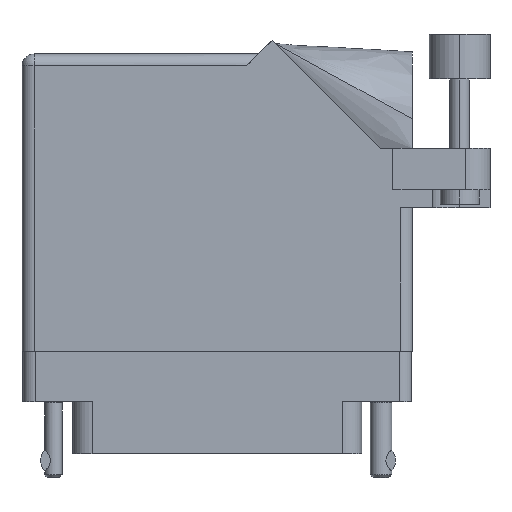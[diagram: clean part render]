
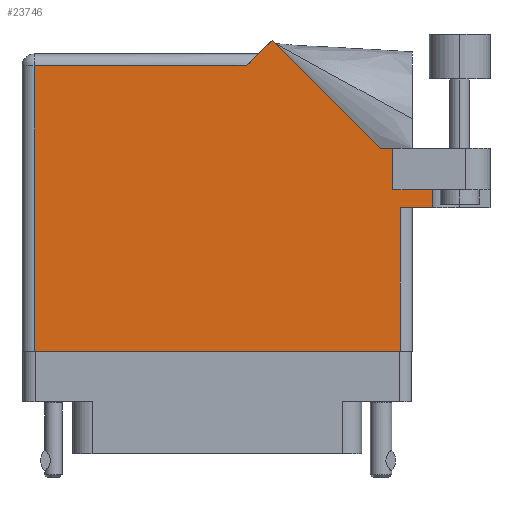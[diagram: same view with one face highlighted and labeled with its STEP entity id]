
A CAD part, front view. The second image highlights one B-rep face of the part: STEP entity #23746.
In plain terms, the highlighted face is planar.
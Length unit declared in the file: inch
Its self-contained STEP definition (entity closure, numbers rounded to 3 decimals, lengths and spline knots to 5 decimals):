
#576 = EDGE_CURVE ( 'NONE', #4813, #48113, #39336, .T. ) ;
#1410 = VERTEX_POINT ( 'NONE', #8539 ) ;
#1434 = CARTESIAN_POINT ( 'NONE',  ( 2.41, 1.044, 0. ) ) ;
#2187 = LINE ( 'NONE', #12493, #23291 ) ;
#2693 = LINE ( 'NONE', #14559, #3306 ) ;
#3215 = ORIENTED_EDGE ( 'NONE', *, *, #45498, .T. ) ;
#3306 = VECTOR ( 'NONE', #48695, 39.37008 ) ;
#4802 = DIRECTION ( 'NONE',  ( -0.707, 0.707, 0. ) ) ;
#4813 = VERTEX_POINT ( 'NONE', #40236 ) ;
#5388 = ORIENTED_EDGE ( 'NONE', *, *, #23080, .T. ) ;
#5591 = VECTOR ( 'NONE', #11149, 39.37008 ) ;
#5718 = EDGE_CURVE ( 'NONE', #39593, #30762, #15890, .T. ) ;
#5849 = VECTOR ( 'NONE', #4802, 39.37008 ) ;
#5967 = VECTOR ( 'NONE', #40439, 39.37008 ) ;
#6289 = VECTOR ( 'NONE', #48000, 39.37008 ) ;
#6350 = CARTESIAN_POINT ( 'NONE',  ( 1.91, 0.831, 0. ) ) ;
#6897 = CARTESIAN_POINT ( 'NONE',  ( 0.062, 0., 0. ) ) ;
#7043 = CARTESIAN_POINT ( 'NONE',  ( 1.155, 1.468, 0. ) ) ;
#8472 = ORIENTED_EDGE ( 'NONE', *, *, #31871, .T. ) ;
#8539 = CARTESIAN_POINT ( 'NONE',  ( 1.948, 0., 0. ) ) ;
#8746 = DIRECTION ( 'NONE',  ( 1., 0., 0. ) ) ;
#10067 = EDGE_CURVE ( 'NONE', #34341, #4813, #33753, .T. ) ;
#11149 = DIRECTION ( 'NONE',  ( -0.707, -0.707, 0. ) ) ;
#12044 = AXIS2_PLACEMENT_3D ( 'NONE', #32890, #40444, #44528 ) ;
#12493 = CARTESIAN_POINT ( 'NONE',  ( 2.01, 0.737, 0. ) ) ;
#12925 = VECTOR ( 'NONE', #42674, 39.37008 ) ;
#13273 = CARTESIAN_POINT ( 'NONE',  ( 1.91, 1.044, 0. ) ) ;
#13551 = ORIENTED_EDGE ( 'NONE', *, *, #17911, .T. ) ;
#14322 = VERTEX_POINT ( 'NONE', #28664 ) ;
#14504 = PLANE ( 'NONE',  #12044 ) ;
#14559 = CARTESIAN_POINT ( 'NONE',  ( 1.91, 0.831, 0. ) ) ;
#15076 = CARTESIAN_POINT ( 'NONE',  ( 1.217, 1.53, 0. ) ) ;
#15890 = LINE ( 'NONE', #47824, #5967 ) ;
#16406 = ORIENTED_EDGE ( 'NONE', *, *, #28903, .F. ) ;
#16605 = ORIENTED_EDGE ( 'NONE', *, *, #576, .T. ) ;
#16777 = LINE ( 'NONE', #6350, #6289 ) ;
#17911 = EDGE_CURVE ( 'NONE', #36560, #1410, #41354, .T. ) ;
#19127 = FACE_OUTER_BOUND ( 'NONE', #48431, .T. ) ;
#20211 = DIRECTION ( 'NONE',  ( 0., 1., 0. ) ) ;
#21383 = LINE ( 'NONE', #15076, #5591 ) ;
#22891 = LINE ( 'NONE', #38447, #12925 ) ;
#23080 = EDGE_CURVE ( 'NONE', #14322, #29942, #2187, .T. ) ;
#23135 = DIRECTION ( 'NONE',  ( 1., 0., 0. ) ) ;
#23290 = CARTESIAN_POINT ( 'NONE',  ( 1.84442, 1.044, 0. ) ) ;
#23291 = VECTOR ( 'NONE', #8746, 39.37008 ) ;
#23734 = VECTOR ( 'NONE', #27661, 39.37008 ) ;
#23746 = ADVANCED_FACE ( 'NONE', ( #19127 ), #14504, .F. ) ;
#24155 = CARTESIAN_POINT ( 'NONE',  ( 1.948, 0.737, 0. ) ) ;
#24202 = CARTESIAN_POINT ( 'NONE',  ( 1.91, 0.831, 0. ) ) ;
#24227 = VECTOR ( 'NONE', #20211, 39.37008 ) ;
#24784 = LINE ( 'NONE', #24155, #24227 ) ;
#25334 = LINE ( 'NONE', #6897, #31227 ) ;
#26130 = CARTESIAN_POINT ( 'NONE',  ( 0.062, 0., 0. ) ) ;
#27011 = CARTESIAN_POINT ( 'NONE',  ( 2.1115, 0.831, 0. ) ) ;
#27661 = DIRECTION ( 'NONE',  ( -1., 0., 0. ) ) ;
#28303 = ORIENTED_EDGE ( 'NONE', *, *, #10067, .T. ) ;
#28664 = CARTESIAN_POINT ( 'NONE',  ( 1.948, 0.737, 0. ) ) ;
#28903 = EDGE_CURVE ( 'NONE', #39726, #29942, #22891, .T. ) ;
#29942 = VERTEX_POINT ( 'NONE', #30492 ) ;
#30272 = CARTESIAN_POINT ( 'NONE',  ( 1.28771, 1.60071, 0. ) ) ;
#30333 = ORIENTED_EDGE ( 'NONE', *, *, #5718, .T. ) ;
#30492 = CARTESIAN_POINT ( 'NONE',  ( 2.1115, 0.737, 0. ) ) ;
#30762 = VERTEX_POINT ( 'NONE', #38525 ) ;
#31227 = VECTOR ( 'NONE', #44133, 39.37008 ) ;
#31871 = EDGE_CURVE ( 'NONE', #30762, #36560, #25334, .T. ) ;
#32890 = CARTESIAN_POINT ( 'NONE',  ( 0., 1.53, 0. ) ) ;
#33437 = ORIENTED_EDGE ( 'NONE', *, *, #45023, .F. ) ;
#33753 = LINE ( 'NONE', #1434, #23734 ) ;
#34341 = VERTEX_POINT ( 'NONE', #13273 ) ;
#34606 = ORIENTED_EDGE ( 'NONE', *, *, #38677, .T. ) ;
#36560 = VERTEX_POINT ( 'NONE', #26130 ) ;
#37190 = EDGE_CURVE ( 'NONE', #48113, #39593, #21383, .T. ) ;
#38447 = CARTESIAN_POINT ( 'NONE',  ( 2.1115, 1.16177, 0. ) ) ;
#38525 = CARTESIAN_POINT ( 'NONE',  ( 0.062, 1.468, 0. ) ) ;
#38677 = EDGE_CURVE ( 'NONE', #1410, #14322, #24784, .T. ) ;
#39336 = LINE ( 'NONE', #23290, #5849 ) ;
#39593 = VERTEX_POINT ( 'NONE', #7043 ) ;
#39726 = VERTEX_POINT ( 'NONE', #27011 ) ;
#39880 = VERTEX_POINT ( 'NONE', #24202 ) ;
#40236 = CARTESIAN_POINT ( 'NONE',  ( 1.84442, 1.044, 0. ) ) ;
#40439 = DIRECTION ( 'NONE',  ( -1., 0., 0. ) ) ;
#40444 = DIRECTION ( 'NONE',  ( 0., 0., -1. ) ) ;
#40668 = ORIENTED_EDGE ( 'NONE', *, *, #37190, .T. ) ;
#41354 = LINE ( 'NONE', #46153, #42532 ) ;
#42532 = VECTOR ( 'NONE', #23135, 39.37008 ) ;
#42674 = DIRECTION ( 'NONE',  ( 0., -1., 0. ) ) ;
#44133 = DIRECTION ( 'NONE',  ( 0., -1., 0. ) ) ;
#44528 = DIRECTION ( 'NONE',  ( -1., 0., 0. ) ) ;
#45023 = EDGE_CURVE ( 'NONE', #39880, #39726, #16777, .T. ) ;
#45498 = EDGE_CURVE ( 'NONE', #39880, #34341, #2693, .T. ) ;
#46153 = CARTESIAN_POINT ( 'NONE',  ( 0., 0., 0. ) ) ;
#47824 = CARTESIAN_POINT ( 'NONE',  ( 0., 1.468, 0. ) ) ;
#48000 = DIRECTION ( 'NONE',  ( 1., 0., 0. ) ) ;
#48113 = VERTEX_POINT ( 'NONE', #30272 ) ;
#48431 = EDGE_LOOP ( 'NONE', ( #13551, #34606, #5388, #16406, #33437, #3215, #28303, #16605, #40668, #30333, #8472 ) ) ;
#48695 = DIRECTION ( 'NONE',  ( 0., 1., 0. ) ) ;
